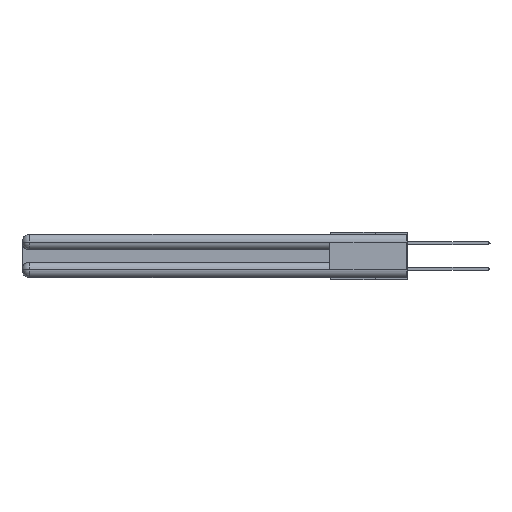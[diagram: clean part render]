
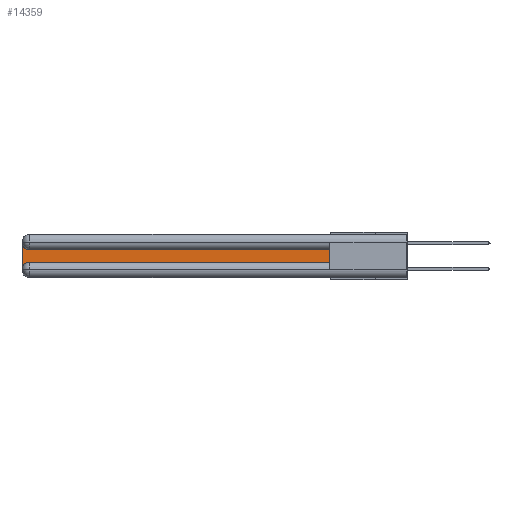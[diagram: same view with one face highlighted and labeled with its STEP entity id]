
A CAD part, left-side view. The second image highlights one B-rep face of the part: STEP entity #14359.
In plain terms, the highlighted planar face has unit normal (-1, 0, 0).
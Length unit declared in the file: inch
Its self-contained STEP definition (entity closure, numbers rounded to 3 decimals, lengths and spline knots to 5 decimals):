
#167 = VERTEX_POINT ( 'NONE', #3031 ) ;
#179 = CARTESIAN_POINT ( 'NONE',  ( 0.075, 0.6, -0.2175 ) ) ;
#836 = EDGE_CURVE ( 'NONE', #167, #31916, #28759, .T. ) ;
#3031 = CARTESIAN_POINT ( 'NONE',  ( 0.075, 0.6, -0.2175 ) ) ;
#3269 = VECTOR ( 'NONE', #9852, 39.37008 ) ;
#3331 = EDGE_LOOP ( 'NONE', ( #6433, #8705, #25757, #5895, #8639, #15523 ) ) ;
#4704 = CARTESIAN_POINT ( 'NONE',  ( 0.075, 2.94, -0.0625 ) ) ;
#5185 = CARTESIAN_POINT ( 'NONE',  ( 0.075, 3., -0.1225 ) ) ;
#5726 = EDGE_CURVE ( 'NONE', #28310, #28909, #12796, .T. ) ;
#5895 = ORIENTED_EDGE ( 'NONE', *, *, #5726, .T. ) ;
#6099 = CARTESIAN_POINT ( 'NONE',  ( 0.075, 0.6, -0.1225 ) ) ;
#6433 = ORIENTED_EDGE ( 'NONE', *, *, #23647, .T. ) ;
#7161 = CARTESIAN_POINT ( 'NONE',  ( 0.075, 0.6, -0.1225 ) ) ;
#8176 = VECTOR ( 'NONE', #21370, 39.37008 ) ;
#8186 = CIRCLE ( 'NONE', #32027, 0.06 ) ;
#8481 = LINE ( 'NONE', #7161, #26994 ) ;
#8639 = ORIENTED_EDGE ( 'NONE', *, *, #28142, .T. ) ;
#8705 = ORIENTED_EDGE ( 'NONE', *, *, #22361, .T. ) ;
#9705 = DIRECTION ( 'NONE',  ( 0., 0., -1. ) ) ;
#9832 = DIRECTION ( 'NONE',  ( 1., 0., 0. ) ) ;
#9852 = DIRECTION ( 'NONE',  ( 0., 0., 1. ) ) ;
#10431 = DIRECTION ( 'NONE',  ( 1., 0., 0. ) ) ;
#10770 = CARTESIAN_POINT ( 'NONE',  ( 0.075, 2.94, -0.2775 ) ) ;
#11021 = LINE ( 'NONE', #179, #8176 ) ;
#12759 = DIRECTION ( 'NONE',  ( 0., 0., -1. ) ) ;
#12796 = CIRCLE ( 'NONE', #31123, 0.06 ) ;
#12921 = VERTEX_POINT ( 'NONE', #33339 ) ;
#13823 = VECTOR ( 'NONE', #9705, 39.37008 ) ;
#14359 = ADVANCED_FACE ( 'NONE', ( #24670 ), #33664, .F. ) ;
#15523 = ORIENTED_EDGE ( 'NONE', *, *, #836, .T. ) ;
#15986 = DIRECTION ( 'NONE',  ( 1., 0., 0. ) ) ;
#16648 = EDGE_CURVE ( 'NONE', #12921, #28310, #22510, .T. ) ;
#17722 = DIRECTION ( 'NONE',  ( 0., 0., -1. ) ) ;
#21370 = DIRECTION ( 'NONE',  ( 0., -1., 0. ) ) ;
#22107 = CARTESIAN_POINT ( 'NONE',  ( 0.075, 2.94, -0.2175 ) ) ;
#22361 = EDGE_CURVE ( 'NONE', #28933, #12921, #8186, .T. ) ;
#22510 = LINE ( 'NONE', #33424, #13823 ) ;
#23275 = DIRECTION ( 'NONE',  ( 0., 1., 0. ) ) ;
#23368 = CARTESIAN_POINT ( 'NONE',  ( 0.075, 0.6, -0.2175 ) ) ;
#23647 = EDGE_CURVE ( 'NONE', #31916, #28933, #8481, .T. ) ;
#24670 = FACE_OUTER_BOUND ( 'NONE', #3331, .T. ) ;
#25757 = ORIENTED_EDGE ( 'NONE', *, *, #16648, .T. ) ;
#26994 = VECTOR ( 'NONE', #23275, 39.37008 ) ;
#27917 = CARTESIAN_POINT ( 'NONE',  ( 0.075, 2.94, -0.1225 ) ) ;
#28142 = EDGE_CURVE ( 'NONE', #28909, #167, #11021, .T. ) ;
#28310 = VERTEX_POINT ( 'NONE', #32288 ) ;
#28759 = LINE ( 'NONE', #23368, #3269 ) ;
#28909 = VERTEX_POINT ( 'NONE', #22107 ) ;
#28933 = VERTEX_POINT ( 'NONE', #27917 ) ;
#30418 = AXIS2_PLACEMENT_3D ( 'NONE', #5185, #10431, #12759 ) ;
#31123 = AXIS2_PLACEMENT_3D ( 'NONE', #10770, #15986, #31540 ) ;
#31540 = DIRECTION ( 'NONE',  ( 0., 0., -1. ) ) ;
#31916 = VERTEX_POINT ( 'NONE', #6099 ) ;
#32027 = AXIS2_PLACEMENT_3D ( 'NONE', #4704, #9832, #17722 ) ;
#32288 = CARTESIAN_POINT ( 'NONE',  ( 0.075, 3., -0.2775 ) ) ;
#33339 = CARTESIAN_POINT ( 'NONE',  ( 0.075, 3., -0.0625 ) ) ;
#33424 = CARTESIAN_POINT ( 'NONE',  ( 0.075, 3., -0.2175 ) ) ;
#33664 = PLANE ( 'NONE',  #30418 ) ;
